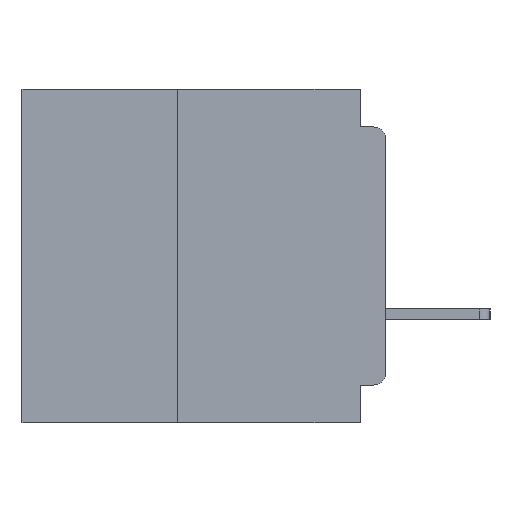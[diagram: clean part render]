
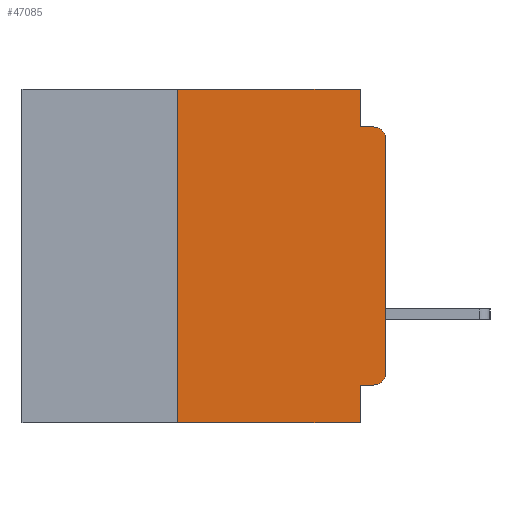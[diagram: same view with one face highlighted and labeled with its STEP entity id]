
A CAD part, left-side view. The second image highlights one B-rep face of the part: STEP entity #47085.
In plain terms, the highlighted planar face has unit normal (-1, 0, 0).
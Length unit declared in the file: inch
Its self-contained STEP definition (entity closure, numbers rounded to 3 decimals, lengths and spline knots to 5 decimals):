
#433 = VECTOR ( 'NONE', #21208, 39.37008 ) ;
#696 = FACE_OUTER_BOUND ( 'NONE', #22010, .T. ) ;
#1059 = VERTEX_POINT ( 'NONE', #59877 ) ;
#1293 = PLANE ( 'NONE',  #11789 ) ;
#3322 = DIRECTION ( 'NONE',  ( 0., 1., 0. ) ) ;
#3966 = VECTOR ( 'NONE', #62337, 39.37008 ) ;
#4172 = DIRECTION ( 'NONE',  ( 0., 0., -1. ) ) ;
#5813 = VECTOR ( 'NONE', #62071, 39.37008 ) ;
#6340 = DIRECTION ( 'NONE',  ( 0., 0., -1. ) ) ;
#6945 = VERTEX_POINT ( 'NONE', #52560 ) ;
#7285 = VECTOR ( 'NONE', #34850, 39.37008 ) ;
#10123 = CARTESIAN_POINT ( 'NONE',  ( 0., 0.437, -0.4 ) ) ;
#11130 = CARTESIAN_POINT ( 'NONE',  ( 0., 0.437, 0. ) ) ;
#11246 = EDGE_CURVE ( 'NONE', #6945, #51275, #15292, .T. ) ;
#11789 = AXIS2_PLACEMENT_3D ( 'NONE', #11130, #36065, #6340 ) ;
#13108 = VERTEX_POINT ( 'NONE', #28449 ) ;
#15292 = LINE ( 'NONE', #50890, #433 ) ;
#17532 = EDGE_CURVE ( 'NONE', #1059, #40833, #35497, .T. ) ;
#19130 = ORIENTED_EDGE ( 'NONE', *, *, #25306, .T. ) ;
#19234 = EDGE_CURVE ( 'NONE', #64006, #13108, #58360, .T. ) ;
#19314 = ORIENTED_EDGE ( 'NONE', *, *, #17532, .T. ) ;
#20513 = DIRECTION ( 'NONE',  ( -1., 0., 0. ) ) ;
#20683 = ORIENTED_EDGE ( 'NONE', *, *, #49811, .F. ) ;
#20860 = ORIENTED_EDGE ( 'NONE', *, *, #62767, .F. ) ;
#20883 = VERTEX_POINT ( 'NONE', #54472 ) ;
#21183 = ORIENTED_EDGE ( 'NONE', *, *, #52876, .F. ) ;
#21208 = DIRECTION ( 'NONE',  ( 0., 0., 1. ) ) ;
#22010 = EDGE_LOOP ( 'NONE', ( #19130, #19314, #20683, #20860, #21183, #22444, #23594, #23783, #24746, #25008 ) ) ;
#22444 = ORIENTED_EDGE ( 'NONE', *, *, #11246, .F. ) ;
#22673 = CARTESIAN_POINT ( 'NONE',  ( 0., 0.031, 0. ) ) ;
#23594 = ORIENTED_EDGE ( 'NONE', *, *, #56989, .T. ) ;
#23783 = ORIENTED_EDGE ( 'NONE', *, *, #51104, .F. ) ;
#23970 = CARTESIAN_POINT ( 'NONE',  ( 0., 0.031, 0. ) ) ;
#24746 = ORIENTED_EDGE ( 'NONE', *, *, #19234, .F. ) ;
#25008 = ORIENTED_EDGE ( 'NONE', *, *, #32847, .T. ) ;
#25306 = EDGE_CURVE ( 'NONE', #43271, #1059, #63480, .T. ) ;
#26779 = LINE ( 'NONE', #22673, #51557 ) ;
#28254 = DIRECTION ( 'NONE',  ( 0., -1., 0. ) ) ;
#28449 = CARTESIAN_POINT ( 'NONE',  ( 0., 0.031, -0.355 ) ) ;
#30817 = DIRECTION ( 'NONE',  ( 0., 0., 1. ) ) ;
#32189 = VECTOR ( 'NONE', #3322, 39.37008 ) ;
#32571 = VERTEX_POINT ( 'NONE', #52804 ) ;
#32636 = CARTESIAN_POINT ( 'NONE',  ( 0., 0., -0.045 ) ) ;
#32847 = EDGE_CURVE ( 'NONE', #64006, #43271, #56966, .T. ) ;
#33732 = LINE ( 'NONE', #10123, #7285 ) ;
#33975 = DIRECTION ( 'NONE',  ( -1., 0., 0. ) ) ;
#34850 = DIRECTION ( 'NONE',  ( 0., -1., 0. ) ) ;
#34921 = LINE ( 'NONE', #57797, #48075 ) ;
#35497 = CIRCLE ( 'NONE', #50318, 0.015 ) ;
#35563 = CARTESIAN_POINT ( 'NONE',  ( 0., 0., 0. ) ) ;
#36031 = CARTESIAN_POINT ( 'NONE',  ( 0., 0., -0.34 ) ) ;
#36065 = DIRECTION ( 'NONE',  ( 1., 0., 0. ) ) ;
#40833 = VERTEX_POINT ( 'NONE', #59336 ) ;
#42423 = DIRECTION ( 'NONE',  ( 0., 0., -1. ) ) ;
#43135 = AXIS2_PLACEMENT_3D ( 'NONE', #50185, #20513, #55106 ) ;
#43271 = VERTEX_POINT ( 'NONE', #36031 ) ;
#43583 = LINE ( 'NONE', #57446, #3966 ) ;
#47085 = ADVANCED_FACE ( 'NONE', ( #696 ), #1293, .F. ) ;
#47823 = CARTESIAN_POINT ( 'NONE',  ( 0., 0., -0.355 ) ) ;
#48075 = VECTOR ( 'NONE', #28254, 39.37008 ) ;
#49384 = VERTEX_POINT ( 'NONE', #23970 ) ;
#49811 = EDGE_CURVE ( 'NONE', #32571, #40833, #56932, .T. ) ;
#50185 = CARTESIAN_POINT ( 'NONE',  ( 0., 0.015, -0.34 ) ) ;
#50318 = AXIS2_PLACEMENT_3D ( 'NONE', #63364, #33975, #4172 ) ;
#50890 = CARTESIAN_POINT ( 'NONE',  ( 0., 0.25, -0.4 ) ) ;
#51104 = EDGE_CURVE ( 'NONE', #13108, #20883, #43583, .T. ) ;
#51275 = VERTEX_POINT ( 'NONE', #54362 ) ;
#51557 = VECTOR ( 'NONE', #42423, 39.37008 ) ;
#52560 = CARTESIAN_POINT ( 'NONE',  ( 0., 0.25, -0.4 ) ) ;
#52804 = CARTESIAN_POINT ( 'NONE',  ( 0., 0.031, -0.045 ) ) ;
#52876 = EDGE_CURVE ( 'NONE', #51275, #49384, #34921, .T. ) ;
#54362 = CARTESIAN_POINT ( 'NONE',  ( 0., 0.25, 0. ) ) ;
#54472 = CARTESIAN_POINT ( 'NONE',  ( 0., 0.031, -0.4 ) ) ;
#55106 = DIRECTION ( 'NONE',  ( 0., 0., -1. ) ) ;
#56932 = LINE ( 'NONE', #32636, #5813 ) ;
#56966 = CIRCLE ( 'NONE', #43135, 0.015 ) ;
#56989 = EDGE_CURVE ( 'NONE', #6945, #20883, #33732, .T. ) ;
#57446 = CARTESIAN_POINT ( 'NONE',  ( 0., 0.031, -0.4 ) ) ;
#57797 = CARTESIAN_POINT ( 'NONE',  ( 0., 0.437, 0. ) ) ;
#57978 = CARTESIAN_POINT ( 'NONE',  ( 0., 0.015, -0.355 ) ) ;
#58360 = LINE ( 'NONE', #47823, #32189 ) ;
#59336 = CARTESIAN_POINT ( 'NONE',  ( 0., 0.015, -0.045 ) ) ;
#59877 = CARTESIAN_POINT ( 'NONE',  ( 0., 0., -0.06 ) ) ;
#60443 = VECTOR ( 'NONE', #30817, 39.37008 ) ;
#62071 = DIRECTION ( 'NONE',  ( 0., -1., 0. ) ) ;
#62337 = DIRECTION ( 'NONE',  ( 0., 0., -1. ) ) ;
#62767 = EDGE_CURVE ( 'NONE', #49384, #32571, #26779, .T. ) ;
#63364 = CARTESIAN_POINT ( 'NONE',  ( 0., 0.015, -0.06 ) ) ;
#63480 = LINE ( 'NONE', #35563, #60443 ) ;
#64006 = VERTEX_POINT ( 'NONE', #57978 ) ;
